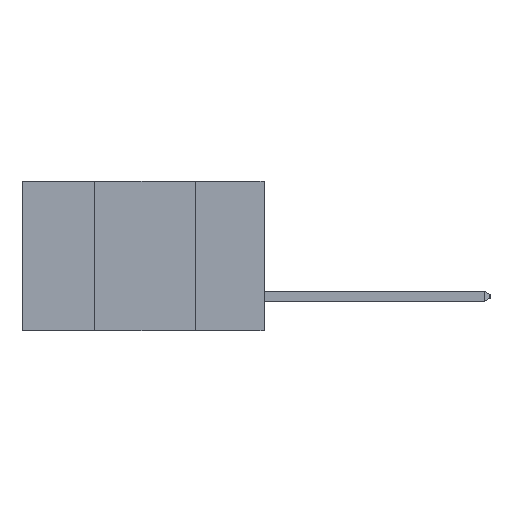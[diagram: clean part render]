
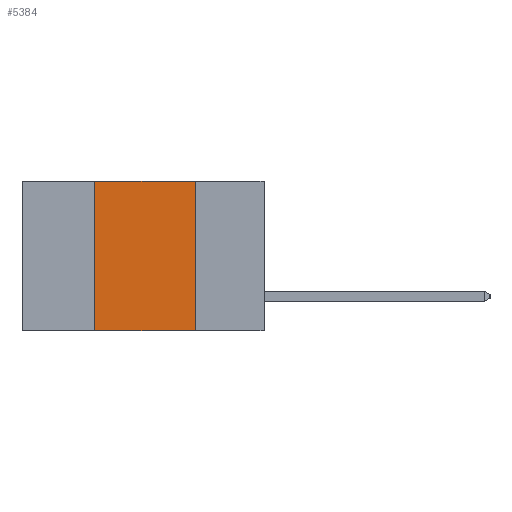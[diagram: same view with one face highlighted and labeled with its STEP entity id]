
A CAD part, left-side view. The second image highlights one B-rep face of the part: STEP entity #5384.
In plain terms, the highlighted planar face has unit normal (-1, 0, 0).
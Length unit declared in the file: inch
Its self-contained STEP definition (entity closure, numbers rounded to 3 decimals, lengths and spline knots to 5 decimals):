
#102 = VERTEX_POINT ( 'NONE', #9401 ) ;
#875 = AXIS2_PLACEMENT_3D ( 'NONE', #8303, #4459, #11273 ) ;
#1410 = VERTEX_POINT ( 'NONE', #7789 ) ;
#1499 = PLANE ( 'NONE',  #875 ) ;
#1832 = LINE ( 'NONE', #8021, #10922 ) ;
#2394 = CARTESIAN_POINT ( 'NONE',  ( 0., 0.17, -0.37 ) ) ;
#2977 = VECTOR ( 'NONE', #11054, 39.37008 ) ;
#2982 = CARTESIAN_POINT ( 'NONE',  ( 0., 0.42, -0.37 ) ) ;
#3345 = FACE_OUTER_BOUND ( 'NONE', #5210, .T. ) ;
#4459 = DIRECTION ( 'NONE',  ( 1., 0., 0. ) ) ;
#5028 = EDGE_CURVE ( 'NONE', #102, #1410, #8379, .T. ) ;
#5210 = EDGE_LOOP ( 'NONE', ( #6316, #8707, #10926, #8961 ) ) ;
#5384 = ADVANCED_FACE ( 'NONE', ( #3345 ), #1499, .F. ) ;
#5957 = VECTOR ( 'NONE', #10942, 39.37008 ) ;
#6316 = ORIENTED_EDGE ( 'NONE', *, *, #5028, .F. ) ;
#6922 = EDGE_CURVE ( 'NONE', #8752, #102, #1832, .T. ) ;
#7138 = VERTEX_POINT ( 'NONE', #2982 ) ;
#7551 = EDGE_CURVE ( 'NONE', #7138, #8752, #7767, .T. ) ;
#7610 = DIRECTION ( 'NONE',  ( 0., -1., 0. ) ) ;
#7767 = LINE ( 'NONE', #10231, #2977 ) ;
#7789 = CARTESIAN_POINT ( 'NONE',  ( 0., 0.17, -0.37 ) ) ;
#8021 = CARTESIAN_POINT ( 'NONE',  ( 0., 0.6, 0. ) ) ;
#8303 = CARTESIAN_POINT ( 'NONE',  ( 0., 0.6, 0. ) ) ;
#8344 = CARTESIAN_POINT ( 'NONE',  ( 0., 0.42, 0. ) ) ;
#8379 = LINE ( 'NONE', #2394, #5957 ) ;
#8707 = ORIENTED_EDGE ( 'NONE', *, *, #6922, .F. ) ;
#8735 = LINE ( 'NONE', #10499, #10691 ) ;
#8752 = VERTEX_POINT ( 'NONE', #8344 ) ;
#8961 = ORIENTED_EDGE ( 'NONE', *, *, #9246, .T. ) ;
#9246 = EDGE_CURVE ( 'NONE', #7138, #1410, #8735, .T. ) ;
#9401 = CARTESIAN_POINT ( 'NONE',  ( 0., 0.17, 0. ) ) ;
#10231 = CARTESIAN_POINT ( 'NONE',  ( 0., 0.42, -0.37 ) ) ;
#10499 = CARTESIAN_POINT ( 'NONE',  ( 0., 0.6, -0.37 ) ) ;
#10691 = VECTOR ( 'NONE', #11311, 39.37008 ) ;
#10922 = VECTOR ( 'NONE', #7610, 39.37008 ) ;
#10926 = ORIENTED_EDGE ( 'NONE', *, *, #7551, .F. ) ;
#10942 = DIRECTION ( 'NONE',  ( 0., 0., -1. ) ) ;
#11054 = DIRECTION ( 'NONE',  ( 0., 0., 1. ) ) ;
#11273 = DIRECTION ( 'NONE',  ( 0., 0., -1. ) ) ;
#11311 = DIRECTION ( 'NONE',  ( 0., -1., 0. ) ) ;
